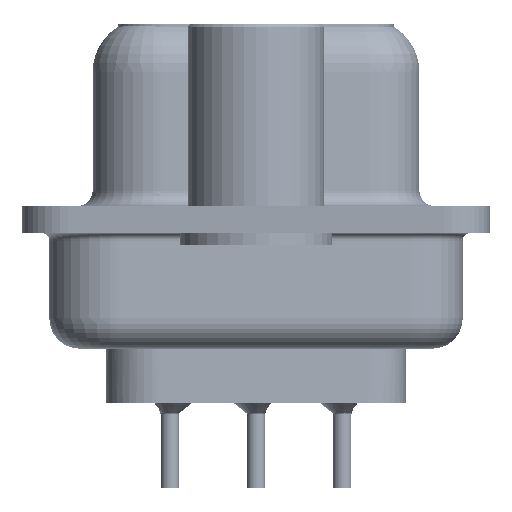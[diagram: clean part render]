
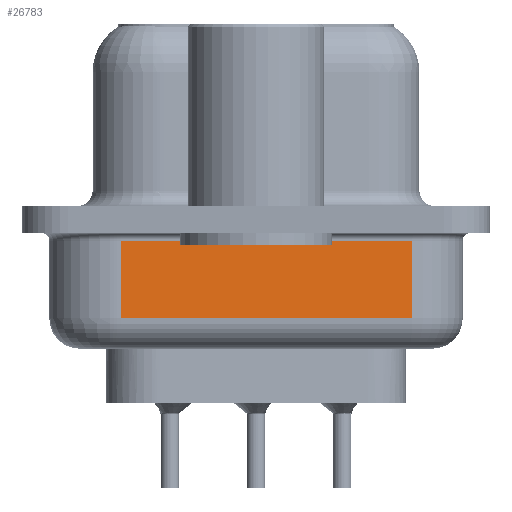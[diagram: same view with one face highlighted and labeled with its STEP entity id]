
A CAD part, left-side view. The second image highlights one B-rep face of the part: STEP entity #26783.
In plain terms, the highlighted planar face has unit normal (-0.985, -0.174, 0).
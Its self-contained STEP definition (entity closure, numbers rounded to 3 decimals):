
#1330 = CARTESIAN_POINT ( 'NONE',  ( 2.93, 4.453, -0.7 ) ) ;
#2192 = VERTEX_POINT ( 'NONE', #1330 ) ;
#3776 = DIRECTION ( 'NONE',  ( 0.985, 0.174, 0. ) ) ;
#3895 = ORIENTED_EDGE ( 'NONE', *, *, #15560, .T. ) ;
#4352 = VECTOR ( 'NONE', #15988, 1000. ) ;
#5341 = DIRECTION ( 'NONE',  ( -0.174, 0.985, 0. ) ) ;
#8279 = DIRECTION ( 'NONE',  ( 0., 0., 1. ) ) ;
#10259 = CARTESIAN_POINT ( 'NONE',  ( 2.93, 4.453, -4.25 ) ) ;
#11210 = LINE ( 'NONE', #12171, #27627 ) ;
#12171 = CARTESIAN_POINT ( 'NONE',  ( 2.93, 4.453, -3.25 ) ) ;
#12314 = ORIENTED_EDGE ( 'NONE', *, *, #24341, .T. ) ;
#15049 = LINE ( 'NONE', #24747, #32443 ) ;
#15508 = DIRECTION ( 'NONE',  ( 0.174, -0.985, 0. ) ) ;
#15560 = EDGE_CURVE ( 'NONE', #23632, #25867, #11210, .T. ) ;
#15988 = DIRECTION ( 'NONE',  ( 0., 0., 1. ) ) ;
#17118 = VECTOR ( 'NONE', #5341, 1000. ) ;
#18139 = LINE ( 'NONE', #28276, #17118 ) ;
#19292 = CARTESIAN_POINT ( 'NONE',  ( 4.623, -5.147, -4.25 ) ) ;
#21198 = CARTESIAN_POINT ( 'NONE',  ( 2.93, 4.453, -3.25 ) ) ;
#23204 = FACE_OUTER_BOUND ( 'NONE', #42581, .T. ) ;
#23466 = PLANE ( 'NONE',  #28808 ) ;
#23632 = VERTEX_POINT ( 'NONE', #21198 ) ;
#23965 = VERTEX_POINT ( 'NONE', #39368 ) ;
#24341 = EDGE_CURVE ( 'NONE', #23965, #2192, #18139, .T. ) ;
#24747 = CARTESIAN_POINT ( 'NONE',  ( 2.93, 4.453, -4.25 ) ) ;
#25867 = VERTEX_POINT ( 'NONE', #41692 ) ;
#26428 = EDGE_CURVE ( 'NONE', #23632, #2192, #15049, .T. ) ;
#26750 = DIRECTION ( 'NONE',  ( -0.174, 0.985, 0. ) ) ;
#26783 = ADVANCED_FACE ( 'NONE', ( #23204 ), #23466, .F. ) ;
#27627 = VECTOR ( 'NONE', #15508, 1000. ) ;
#28276 = CARTESIAN_POINT ( 'NONE',  ( 2.93, 4.453, -0.7 ) ) ;
#28808 = AXIS2_PLACEMENT_3D ( 'NONE', #10259, #3776, #26750 ) ;
#32443 = VECTOR ( 'NONE', #8279, 1000. ) ;
#34570 = ORIENTED_EDGE ( 'NONE', *, *, #26428, .F. ) ;
#35690 = ORIENTED_EDGE ( 'NONE', *, *, #40181, .T. ) ;
#39265 = LINE ( 'NONE', #19292, #4352 ) ;
#39368 = CARTESIAN_POINT ( 'NONE',  ( 4.623, -5.147, -0.7 ) ) ;
#40181 = EDGE_CURVE ( 'NONE', #25867, #23965, #39265, .T. ) ;
#41692 = CARTESIAN_POINT ( 'NONE',  ( 4.623, -5.147, -3.25 ) ) ;
#42581 = EDGE_LOOP ( 'NONE', ( #34570, #3895, #35690, #12314 ) ) ;
